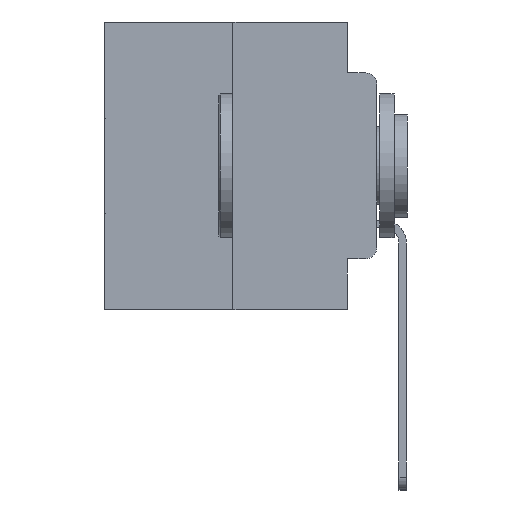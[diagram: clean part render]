
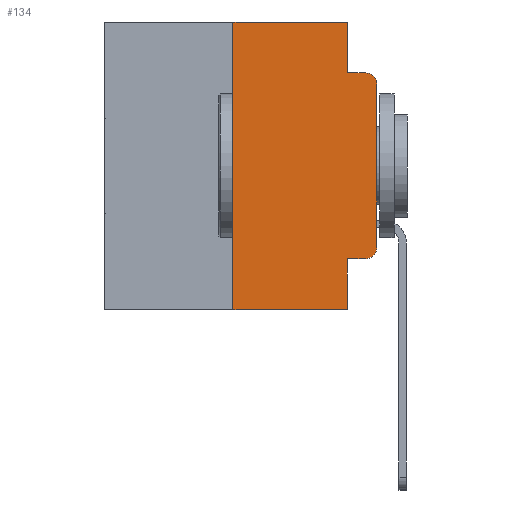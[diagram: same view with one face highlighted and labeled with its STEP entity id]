
A CAD part, left-side view. The second image highlights one B-rep face of the part: STEP entity #134.
In plain terms, the highlighted planar face has unit normal (-1, 0, 0).
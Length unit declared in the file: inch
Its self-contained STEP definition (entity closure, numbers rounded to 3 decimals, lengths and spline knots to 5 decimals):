
#134 = ADVANCED_FACE ( 'NONE', ( #19388 ), #18648, .F. ) ;
#317 = ORIENTED_EDGE ( 'NONE', *, *, #11611, .T. ) ;
#815 = ORIENTED_EDGE ( 'NONE', *, *, #1438, .T. ) ;
#1278 = EDGE_LOOP ( 'NONE', ( #15419, #317, #19755, #28094, #7001, #26191, #16414, #17793, #815, #14028 ) ) ;
#1315 = VECTOR ( 'NONE', #1924, 39.37008 ) ;
#1438 = EDGE_CURVE ( 'NONE', #13552, #14881, #22489, .T. ) ;
#1924 = DIRECTION ( 'NONE',  ( 0., 0., 1. ) ) ;
#2434 = VECTOR ( 'NONE', #4881, 39.37008 ) ;
#2442 = DIRECTION ( 'NONE',  ( 0., -1., 0. ) ) ;
#2571 = LINE ( 'NONE', #9709, #19898 ) ;
#2987 = DIRECTION ( 'NONE',  ( -1., 0., 0. ) ) ;
#3228 = EDGE_CURVE ( 'NONE', #13552, #21509, #2571, .T. ) ;
#4773 = CIRCLE ( 'NONE', #11222, 0.02 ) ;
#4855 = DIRECTION ( 'NONE',  ( 0., -1., 0. ) ) ;
#4881 = DIRECTION ( 'NONE',  ( 0., -1., 0. ) ) ;
#5014 = EDGE_CURVE ( 'NONE', #18898, #27173, #26616, .T. ) ;
#5355 = LINE ( 'NONE', #11113, #16372 ) ;
#5591 = CARTESIAN_POINT ( 'NONE',  ( 0., 0.02, -0.1085 ) ) ;
#5652 = LINE ( 'NONE', #7693, #11400 ) ;
#5873 = CARTESIAN_POINT ( 'NONE',  ( 0., 0., -0.1085 ) ) ;
#6328 = VERTEX_POINT ( 'NONE', #18603 ) ;
#6522 = DIRECTION ( 'NONE',  ( 0., 0., -1. ) ) ;
#6600 = DIRECTION ( 'NONE',  ( 1., 0., 0. ) ) ;
#6758 = EDGE_CURVE ( 'NONE', #6328, #20848, #22861, .T. ) ;
#6786 = CARTESIAN_POINT ( 'NONE',  ( 0., 0.473, 0. ) ) ;
#7001 = ORIENTED_EDGE ( 'NONE', *, *, #24979, .F. ) ;
#7275 = DIRECTION ( 'NONE',  ( 0., 0., -1. ) ) ;
#7693 = CARTESIAN_POINT ( 'NONE',  ( 0., 0.051, -0.0885 ) ) ;
#7877 = CARTESIAN_POINT ( 'NONE',  ( 0., 0.051, -0.5 ) ) ;
#8121 = DIRECTION ( 'NONE',  ( 0., 0., -1. ) ) ;
#9709 = CARTESIAN_POINT ( 'NONE',  ( 0., 0.051, 0. ) ) ;
#9997 = CARTESIAN_POINT ( 'NONE',  ( 0., 0.473, -0.5 ) ) ;
#10108 = EDGE_CURVE ( 'NONE', #20848, #11410, #5652, .T. ) ;
#11113 = CARTESIAN_POINT ( 'NONE',  ( 0., 0., 0. ) ) ;
#11139 = CARTESIAN_POINT ( 'NONE',  ( 0., 0., -0.3915 ) ) ;
#11222 = AXIS2_PLACEMENT_3D ( 'NONE', #17239, #2987, #19432 ) ;
#11400 = VECTOR ( 'NONE', #2442, 39.37008 ) ;
#11410 = VERTEX_POINT ( 'NONE', #18940 ) ;
#11611 = EDGE_CURVE ( 'NONE', #12952, #11410, #17114, .T. ) ;
#11985 = DIRECTION ( 'NONE',  ( 0., 0., -1. ) ) ;
#12300 = VERTEX_POINT ( 'NONE', #11139 ) ;
#12522 = VECTOR ( 'NONE', #22540, 39.37008 ) ;
#12929 = AXIS2_PLACEMENT_3D ( 'NONE', #5591, #21551, #8121 ) ;
#12952 = VERTEX_POINT ( 'NONE', #5873 ) ;
#13115 = EDGE_CURVE ( 'NONE', #12300, #12952, #5355, .T. ) ;
#13552 = VERTEX_POINT ( 'NONE', #29382 ) ;
#14028 = ORIENTED_EDGE ( 'NONE', *, *, #28127, .T. ) ;
#14597 = CARTESIAN_POINT ( 'NONE',  ( 0., 0.25, -0.5 ) ) ;
#14881 = VERTEX_POINT ( 'NONE', #15540 ) ;
#15419 = ORIENTED_EDGE ( 'NONE', *, *, #13115, .T. ) ;
#15540 = CARTESIAN_POINT ( 'NONE',  ( 0., 0.02, -0.4115 ) ) ;
#16372 = VECTOR ( 'NONE', #28470, 39.37008 ) ;
#16414 = ORIENTED_EDGE ( 'NONE', *, *, #24233, .T. ) ;
#17114 = CIRCLE ( 'NONE', #12929, 0.02 ) ;
#17239 = CARTESIAN_POINT ( 'NONE',  ( 0., 0.02, -0.3915 ) ) ;
#17793 = ORIENTED_EDGE ( 'NONE', *, *, #3228, .F. ) ;
#18603 = CARTESIAN_POINT ( 'NONE',  ( 0., 0.051, 0. ) ) ;
#18631 = CARTESIAN_POINT ( 'NONE',  ( 0., 0.25, 0. ) ) ;
#18648 = PLANE ( 'NONE',  #27897 ) ;
#18898 = VERTEX_POINT ( 'NONE', #14597 ) ;
#18940 = CARTESIAN_POINT ( 'NONE',  ( 0., 0.02, -0.0885 ) ) ;
#19365 = CARTESIAN_POINT ( 'NONE',  ( 0., 0.25, 0. ) ) ;
#19388 = FACE_OUTER_BOUND ( 'NONE', #1278, .T. ) ;
#19432 = DIRECTION ( 'NONE',  ( 0., 0., -1. ) ) ;
#19755 = ORIENTED_EDGE ( 'NONE', *, *, #10108, .F. ) ;
#19876 = CARTESIAN_POINT ( 'NONE',  ( 0., 0.051, -0.4115 ) ) ;
#19898 = VECTOR ( 'NONE', #7275, 39.37008 ) ;
#20848 = VERTEX_POINT ( 'NONE', #27773 ) ;
#21509 = VERTEX_POINT ( 'NONE', #7877 ) ;
#21551 = DIRECTION ( 'NONE',  ( -1., 0., 0. ) ) ;
#21782 = LINE ( 'NONE', #9997, #2434 ) ;
#22015 = CARTESIAN_POINT ( 'NONE',  ( 0., 0.473, 0. ) ) ;
#22197 = VECTOR ( 'NONE', #11985, 39.37008 ) ;
#22489 = LINE ( 'NONE', #19876, #27506 ) ;
#22540 = DIRECTION ( 'NONE',  ( 0., -1., 0. ) ) ;
#22861 = LINE ( 'NONE', #27166, #22197 ) ;
#24233 = EDGE_CURVE ( 'NONE', #18898, #21509, #21782, .T. ) ;
#24979 = EDGE_CURVE ( 'NONE', #27173, #6328, #25454, .T. ) ;
#25454 = LINE ( 'NONE', #6786, #12522 ) ;
#26191 = ORIENTED_EDGE ( 'NONE', *, *, #5014, .F. ) ;
#26616 = LINE ( 'NONE', #18631, #1315 ) ;
#27166 = CARTESIAN_POINT ( 'NONE',  ( 0., 0.051, 0. ) ) ;
#27173 = VERTEX_POINT ( 'NONE', #19365 ) ;
#27506 = VECTOR ( 'NONE', #4855, 39.37008 ) ;
#27773 = CARTESIAN_POINT ( 'NONE',  ( 0., 0.051, -0.0885 ) ) ;
#27897 = AXIS2_PLACEMENT_3D ( 'NONE', #22015, #6600, #6522 ) ;
#28094 = ORIENTED_EDGE ( 'NONE', *, *, #6758, .F. ) ;
#28127 = EDGE_CURVE ( 'NONE', #14881, #12300, #4773, .T. ) ;
#28470 = DIRECTION ( 'NONE',  ( 0., 0., 1. ) ) ;
#29382 = CARTESIAN_POINT ( 'NONE',  ( 0., 0.051, -0.4115 ) ) ;
